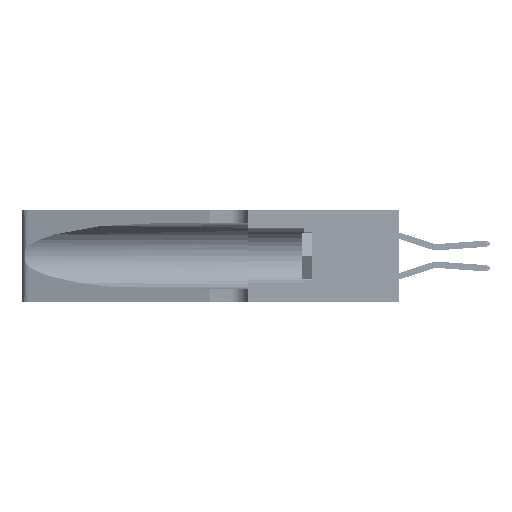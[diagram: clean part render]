
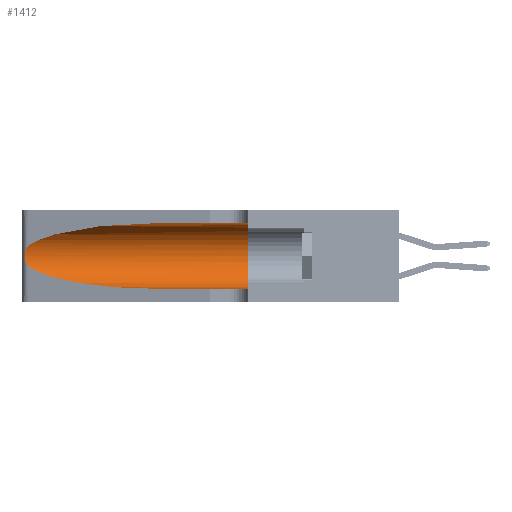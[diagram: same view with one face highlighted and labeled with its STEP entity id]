
A CAD part, left-side view. The second image highlights one B-rep face of the part: STEP entity #1412.
In plain terms, the highlighted cylindrical face has radius 3.308 mm (diameter 6.617 mm), a partial arc.
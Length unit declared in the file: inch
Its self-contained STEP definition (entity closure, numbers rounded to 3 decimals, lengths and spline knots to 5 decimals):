
#1412 = ADVANCED_FACE ( 'NONE', ( #10098 ), #29724, .F. ) ;
#2087 = CARTESIAN_POINT ( 'NONE',  ( 0.1305, 1.61858, 0.05475 ) ) ;
#2682 = CARTESIAN_POINT ( 'NONE',  ( 0.25487, 1.22718, 0.22369 ) ) ;
#3246 = CARTESIAN_POINT ( 'NONE',  ( 0.25487, 1.22718, 0.14631 ) ) ;
#3333 = CARTESIAN_POINT ( 'NONE',  ( 0.25787, 1.23484, 0.2124 ) ) ;
#4295 = CARTESIAN_POINT ( 'NONE',  ( 0.1305, 0.35, 0.31525 ) ) ;
#5072 = EDGE_CURVE ( 'NONE', #31077, #26971, #33682, .T. ) ;
#5819 = CARTESIAN_POINT ( 'NONE',  ( 0.1305, 1.61858, 0.31525 ) ) ;
#5889 = CIRCLE ( 'NONE', #10412, 0.13025 ) ;
#6506 =( BOUNDED_CURVE ( )  B_SPLINE_CURVE ( 3, ( #14450, #37898, #26276, #2682 ),
 .UNSPECIFIED., .F., .T. ) 
 B_SPLINE_CURVE_WITH_KNOTS ( ( 4, 4 ),
 ( 1.5708, 2.84003 ),
 .UNSPECIFIED. ) 
 CURVE ( )  GEOMETRIC_REPRESENTATION_ITEM ( )  RATIONAL_B_SPLINE_CURVE ( ( 1., 0.87, 0.87, 1. ) ) 
 REPRESENTATION_ITEM ( '' )  );
#7336 = CARTESIAN_POINT ( 'NONE',  ( 0.26018, 1.23835, 0.19895 ) ) ;
#8282 = CARTESIAN_POINT ( 'NONE',  ( 0.18966, 0.96281, 0.05475 ) ) ;
#9830 = DIRECTION ( 'NONE',  ( 0., -1., 0. ) ) ;
#10098 = FACE_OUTER_BOUND ( 'NONE', #18972, .T. ) ;
#10412 = AXIS2_PLACEMENT_3D ( 'NONE', #40148, #16696, #44033 ) ;
#11283 = CARTESIAN_POINT ( 'NONE',  ( 0.26075, 1.23896, 0.178 ) ) ;
#13773 = CARTESIAN_POINT ( 'NONE',  ( 0.1305, 1.61858, 0.185 ) ) ;
#14450 = CARTESIAN_POINT ( 'NONE',  ( 0.1305, 0.72297, 0.31525 ) ) ;
#15243 = CARTESIAN_POINT ( 'NONE',  ( 0.25856, 1.23593, 0.16098 ) ) ;
#15627 = B_SPLINE_CURVE_WITH_KNOTS ( 'NONE', 3,
 ( #26903, #50219, #19001, #3333, #30817, #7336, #34738, #11283, #38656, #15243, #42595, #19172, #46499, #23113 ),
 .UNSPECIFIED., .F., .F.,
 ( 4, 2, 2, 2, 2, 2, 4 ),
 ( 0., 0.00027, 0.00053, 0.00107, 0.0016, 0.00187, 0.00214 ),
 .UNSPECIFIED. ) ;
#16696 = DIRECTION ( 'NONE',  ( 0., 1., 0. ) ) ;
#18009 = DIRECTION ( 'NONE',  ( 0., -1., 0. ) ) ;
#18972 = EDGE_LOOP ( 'NONE', ( #32711, #32638, #25105, #23299, #45460, #42346 ) ) ;
#19001 = CARTESIAN_POINT ( 'NONE',  ( 0.25639, 1.23184, 0.21858 ) ) ;
#19172 = CARTESIAN_POINT ( 'NONE',  ( 0.25639, 1.23186, 0.15144 ) ) ;
#19607 = EDGE_CURVE ( 'NONE', #43077, #35824, #15627, .T. ) ;
#22064 = VECTOR ( 'NONE', #39414, 39.37008 ) ;
#23113 = CARTESIAN_POINT ( 'NONE',  ( 0.25487, 1.22718, 0.14631 ) ) ;
#23253 = AXIS2_PLACEMENT_3D ( 'NONE', #13773, #9830, #37224 ) ;
#23299 = ORIENTED_EDGE ( 'NONE', *, *, #49124, .T. ) ;
#23864 = CARTESIAN_POINT ( 'NONE',  ( 0.25487, 1.22718, 0.14631 ) ) ;
#23892 = CARTESIAN_POINT ( 'NONE',  ( 0.25487, 1.22718, 0.22369 ) ) ;
#24498 = EDGE_CURVE ( 'NONE', #26971, #48966, #5889, .T. ) ;
#24796 = EDGE_CURVE ( 'NONE', #31077, #43077, #6506, .T. ) ;
#25025 = EDGE_CURVE ( 'NONE', #35824, #42372, #48179, .T. ) ;
#25105 = ORIENTED_EDGE ( 'NONE', *, *, #25025, .T. ) ;
#26276 = CARTESIAN_POINT ( 'NONE',  ( 0.2373, 1.15595, 0.28018 ) ) ;
#26903 = CARTESIAN_POINT ( 'NONE',  ( 0.25487, 1.22718, 0.22369 ) ) ;
#26971 = VERTEX_POINT ( 'NONE', #4295 ) ;
#29724 = CYLINDRICAL_SURFACE ( 'NONE', #23253, 0.13025 ) ;
#30817 = CARTESIAN_POINT ( 'NONE',  ( 0.25854, 1.2359, 0.20912 ) ) ;
#31077 = VERTEX_POINT ( 'NONE', #46394 ) ;
#32638 = ORIENTED_EDGE ( 'NONE', *, *, #19607, .T. ) ;
#32711 = ORIENTED_EDGE ( 'NONE', *, *, #24796, .T. ) ;
#32737 = CARTESIAN_POINT ( 'NONE',  ( 0.1305, 0.35, 0.05475 ) ) ;
#33682 = LINE ( 'NONE', #5819, #22064 ) ;
#34738 = CARTESIAN_POINT ( 'NONE',  ( 0.26075, 1.23896, 0.19203 ) ) ;
#35118 = VECTOR ( 'NONE', #18009, 39.37008 ) ;
#35665 = CARTESIAN_POINT ( 'NONE',  ( 0.1305, 0.72297, 0.05475 ) ) ;
#35824 = VERTEX_POINT ( 'NONE', #3246 ) ;
#36363 = LINE ( 'NONE', #2087, #35118 ) ;
#37224 = DIRECTION ( 'NONE',  ( 0., 0., -1. ) ) ;
#37898 = CARTESIAN_POINT ( 'NONE',  ( 0.18966, 0.96281, 0.31525 ) ) ;
#38656 = CARTESIAN_POINT ( 'NONE',  ( 0.26017, 1.23833, 0.17102 ) ) ;
#39414 = DIRECTION ( 'NONE',  ( 0., -1., 0. ) ) ;
#39418 = CARTESIAN_POINT ( 'NONE',  ( 0.2373, 1.15595, 0.08982 ) ) ;
#40148 = CARTESIAN_POINT ( 'NONE',  ( 0.1305, 0.35, 0.185 ) ) ;
#42346 = ORIENTED_EDGE ( 'NONE', *, *, #5072, .F. ) ;
#42372 = VERTEX_POINT ( 'NONE', #47334 ) ;
#42595 = CARTESIAN_POINT ( 'NONE',  ( 0.25789, 1.23486, 0.15765 ) ) ;
#43077 = VERTEX_POINT ( 'NONE', #23892 ) ;
#44033 = DIRECTION ( 'NONE',  ( 0., 0., 1. ) ) ;
#45460 = ORIENTED_EDGE ( 'NONE', *, *, #24498, .F. ) ;
#46394 = CARTESIAN_POINT ( 'NONE',  ( 0.1305, 0.72297, 0.31525 ) ) ;
#46499 = CARTESIAN_POINT ( 'NONE',  ( 0.25555, 1.22993, 0.14849 ) ) ;
#47334 = CARTESIAN_POINT ( 'NONE',  ( 0.1305, 0.72297, 0.05475 ) ) ;
#48179 =( BOUNDED_CURVE ( )  B_SPLINE_CURVE ( 3, ( #23864, #39418, #8282, #35665 ),
 .UNSPECIFIED., .F., .F. ) 
 B_SPLINE_CURVE_WITH_KNOTS ( ( 4, 4 ),
 ( 3.44316, 4.71239 ),
 .UNSPECIFIED. ) 
 CURVE ( )  GEOMETRIC_REPRESENTATION_ITEM ( )  RATIONAL_B_SPLINE_CURVE ( ( 1., 0.87, 0.87, 1. ) ) 
 REPRESENTATION_ITEM ( '' )  );
#48966 = VERTEX_POINT ( 'NONE', #32737 ) ;
#49124 = EDGE_CURVE ( 'NONE', #42372, #48966, #36363, .T. ) ;
#50219 = CARTESIAN_POINT ( 'NONE',  ( 0.25555, 1.22994, 0.2215 ) ) ;
